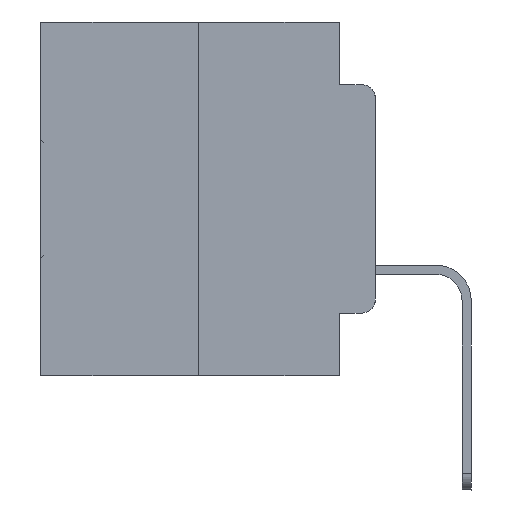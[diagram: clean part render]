
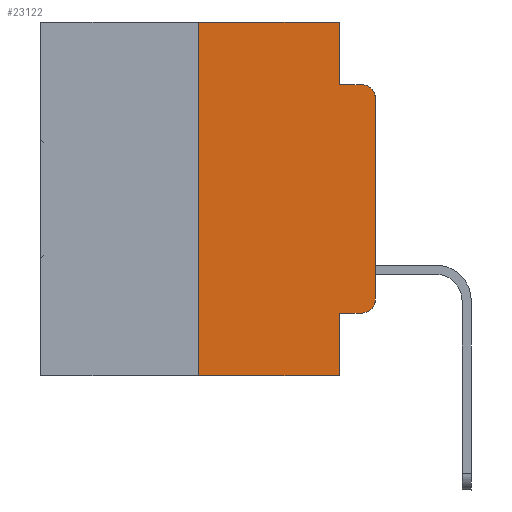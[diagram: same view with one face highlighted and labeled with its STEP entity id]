
A CAD part, left-side view. The second image highlights one B-rep face of the part: STEP entity #23122.
In plain terms, the highlighted planar face has unit normal (-1, 0, 0).
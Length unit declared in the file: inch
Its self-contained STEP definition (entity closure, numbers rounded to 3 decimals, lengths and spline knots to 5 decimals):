
#157 = DIRECTION ( 'NONE',  ( 0., 0., -1. ) ) ;
#191 = VERTEX_POINT ( 'NONE', #3726 ) ;
#1003 = CARTESIAN_POINT ( 'NONE',  ( 0., 0.473, 0. ) ) ;
#1277 = PLANE ( 'NONE',  #13613 ) ;
#1447 = VECTOR ( 'NONE', #9638, 39.37008 ) ;
#1771 = ORIENTED_EDGE ( 'NONE', *, *, #4377, .T. ) ;
#2121 = EDGE_CURVE ( 'NONE', #15516, #17155, #14821, .T. ) ;
#2184 = LINE ( 'NONE', #23967, #1447 ) ;
#2291 = ORIENTED_EDGE ( 'NONE', *, *, #14909, .T. ) ;
#2338 = DIRECTION ( 'NONE',  ( 0., -1., 0. ) ) ;
#2938 = VECTOR ( 'NONE', #2338, 39.37008 ) ;
#3007 = EDGE_CURVE ( 'NONE', #24499, #27994, #26963, .T. ) ;
#3209 = CARTESIAN_POINT ( 'NONE',  ( 0., 0.25, 0. ) ) ;
#3249 = VERTEX_POINT ( 'NONE', #29080 ) ;
#3355 = DIRECTION ( 'NONE',  ( 0., 0., -1. ) ) ;
#3423 = EDGE_CURVE ( 'NONE', #7125, #3249, #16199, .T. ) ;
#3454 = ORIENTED_EDGE ( 'NONE', *, *, #16256, .T. ) ;
#3726 = CARTESIAN_POINT ( 'NONE',  ( 0., 0., -0.3915 ) ) ;
#4227 = CARTESIAN_POINT ( 'NONE',  ( 0., 0.051, -0.0885 ) ) ;
#4377 = EDGE_CURVE ( 'NONE', #191, #4473, #16118, .T. ) ;
#4473 = VERTEX_POINT ( 'NONE', #19830 ) ;
#5486 = ORIENTED_EDGE ( 'NONE', *, *, #2121, .F. ) ;
#6314 = VECTOR ( 'NONE', #7855, 39.37008 ) ;
#7125 = VERTEX_POINT ( 'NONE', #28279 ) ;
#7157 = EDGE_LOOP ( 'NONE', ( #1771, #22970, #21498, #11622, #5486, #19549, #3454, #29309, #23791, #2291 ) ) ;
#7364 = CARTESIAN_POINT ( 'NONE',  ( 0., 0.051, -0.4115 ) ) ;
#7725 = VECTOR ( 'NONE', #16543, 39.37008 ) ;
#7855 = DIRECTION ( 'NONE',  ( 0., -1., 0. ) ) ;
#9556 = VECTOR ( 'NONE', #10363, 39.37008 ) ;
#9638 = DIRECTION ( 'NONE',  ( 0., 0., -1. ) ) ;
#9851 = CARTESIAN_POINT ( 'NONE',  ( 0., 0.02, -0.3915 ) ) ;
#10081 = DIRECTION ( 'NONE',  ( -1., 0., 0. ) ) ;
#10169 = CARTESIAN_POINT ( 'NONE',  ( 0., 0.02, -0.0885 ) ) ;
#10363 = DIRECTION ( 'NONE',  ( 0., 0., 1. ) ) ;
#10468 = VERTEX_POINT ( 'NONE', #15936 ) ;
#10789 = DIRECTION ( 'NONE',  ( 1., 0., 0. ) ) ;
#11120 = EDGE_CURVE ( 'NONE', #17155, #24499, #29645, .T. ) ;
#11180 = AXIS2_PLACEMENT_3D ( 'NONE', #9851, #28971, #19250 ) ;
#11337 = VECTOR ( 'NONE', #26325, 39.37008 ) ;
#11622 = ORIENTED_EDGE ( 'NONE', *, *, #11120, .F. ) ;
#12058 = CARTESIAN_POINT ( 'NONE',  ( 0., 0.02, -0.1085 ) ) ;
#13613 = AXIS2_PLACEMENT_3D ( 'NONE', #15139, #10789, #3355 ) ;
#13743 = CARTESIAN_POINT ( 'NONE',  ( 0., 0.051, 0. ) ) ;
#13846 = DIRECTION ( 'NONE',  ( 0., -1., 0. ) ) ;
#14361 = EDGE_CURVE ( 'NONE', #4473, #27994, #27130, .T. ) ;
#14821 = LINE ( 'NONE', #1003, #6314 ) ;
#14909 = EDGE_CURVE ( 'NONE', #3249, #191, #28954, .T. ) ;
#15139 = CARTESIAN_POINT ( 'NONE',  ( 0., 0.473, 0. ) ) ;
#15516 = VERTEX_POINT ( 'NONE', #29907 ) ;
#15936 = CARTESIAN_POINT ( 'NONE',  ( 0., 0.051, -0.5 ) ) ;
#16118 = LINE ( 'NONE', #23943, #11337 ) ;
#16199 = LINE ( 'NONE', #7364, #7725 ) ;
#16256 = EDGE_CURVE ( 'NONE', #19636, #10468, #21084, .T. ) ;
#16505 = CARTESIAN_POINT ( 'NONE',  ( 0., 0.051, -0.0885 ) ) ;
#16543 = DIRECTION ( 'NONE',  ( 0., -1., 0. ) ) ;
#17155 = VERTEX_POINT ( 'NONE', #26889 ) ;
#18491 = DIRECTION ( 'NONE',  ( 0., 0., -1. ) ) ;
#19250 = DIRECTION ( 'NONE',  ( 0., 0., -1. ) ) ;
#19549 = ORIENTED_EDGE ( 'NONE', *, *, #25670, .F. ) ;
#19636 = VERTEX_POINT ( 'NONE', #26153 ) ;
#19830 = CARTESIAN_POINT ( 'NONE',  ( 0., 0., -0.1085 ) ) ;
#21084 = LINE ( 'NONE', #23632, #29972 ) ;
#21425 = AXIS2_PLACEMENT_3D ( 'NONE', #12058, #10081, #157 ) ;
#21498 = ORIENTED_EDGE ( 'NONE', *, *, #3007, .F. ) ;
#22848 = FACE_OUTER_BOUND ( 'NONE', #7157, .T. ) ;
#22970 = ORIENTED_EDGE ( 'NONE', *, *, #14361, .T. ) ;
#23122 = ADVANCED_FACE ( 'NONE', ( #22848 ), #1277, .F. ) ;
#23601 = LINE ( 'NONE', #3209, #9556 ) ;
#23632 = CARTESIAN_POINT ( 'NONE',  ( 0., 0.473, -0.5 ) ) ;
#23791 = ORIENTED_EDGE ( 'NONE', *, *, #3423, .T. ) ;
#23943 = CARTESIAN_POINT ( 'NONE',  ( 0., 0., 0. ) ) ;
#23967 = CARTESIAN_POINT ( 'NONE',  ( 0., 0.051, 0. ) ) ;
#24499 = VERTEX_POINT ( 'NONE', #4227 ) ;
#25493 = EDGE_CURVE ( 'NONE', #7125, #10468, #2184, .T. ) ;
#25670 = EDGE_CURVE ( 'NONE', #19636, #15516, #23601, .T. ) ;
#26153 = CARTESIAN_POINT ( 'NONE',  ( 0., 0.25, -0.5 ) ) ;
#26325 = DIRECTION ( 'NONE',  ( 0., 0., 1. ) ) ;
#26889 = CARTESIAN_POINT ( 'NONE',  ( 0., 0.051, 0. ) ) ;
#26963 = LINE ( 'NONE', #16505, #2938 ) ;
#27050 = VECTOR ( 'NONE', #18491, 39.37008 ) ;
#27130 = CIRCLE ( 'NONE', #21425, 0.02 ) ;
#27994 = VERTEX_POINT ( 'NONE', #10169 ) ;
#28279 = CARTESIAN_POINT ( 'NONE',  ( 0., 0.051, -0.4115 ) ) ;
#28954 = CIRCLE ( 'NONE', #11180, 0.02 ) ;
#28971 = DIRECTION ( 'NONE',  ( -1., 0., 0. ) ) ;
#29080 = CARTESIAN_POINT ( 'NONE',  ( 0., 0.02, -0.4115 ) ) ;
#29309 = ORIENTED_EDGE ( 'NONE', *, *, #25493, .F. ) ;
#29645 = LINE ( 'NONE', #13743, #27050 ) ;
#29907 = CARTESIAN_POINT ( 'NONE',  ( 0., 0.25, 0. ) ) ;
#29972 = VECTOR ( 'NONE', #13846, 39.37008 ) ;
